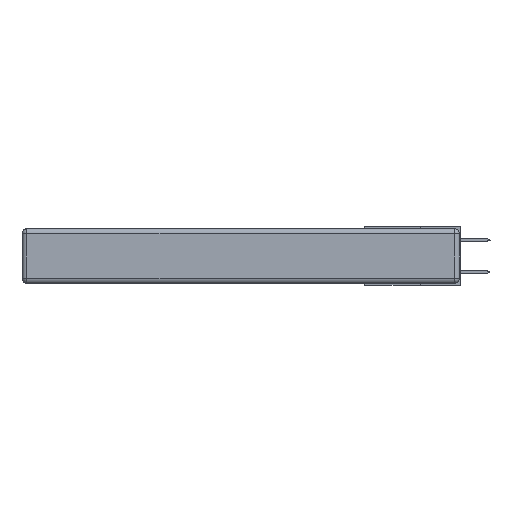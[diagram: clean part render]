
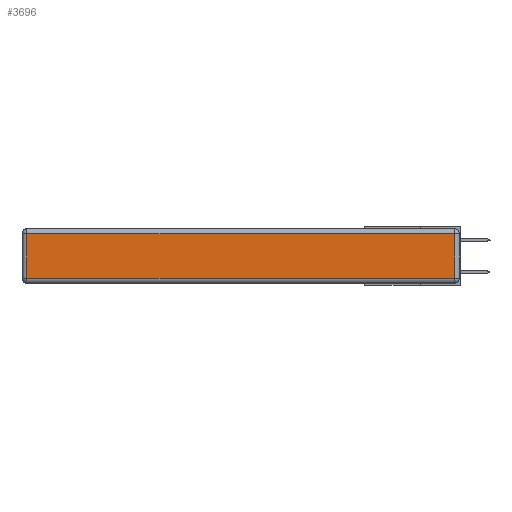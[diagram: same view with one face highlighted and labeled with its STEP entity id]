
A CAD part, left-side view. The second image highlights one B-rep face of the part: STEP entity #3696.
In plain terms, the highlighted planar face has unit normal (-1, 0, 0).
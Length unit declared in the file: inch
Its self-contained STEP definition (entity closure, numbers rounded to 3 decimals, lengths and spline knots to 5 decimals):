
#923 = ORIENTED_EDGE ( 'NONE', *, *, #18820, .T. ) ;
#1797 = EDGE_CURVE ( 'NONE', #11398, #5262, #14673, .T. ) ;
#3696 = ADVANCED_FACE ( 'NONE', ( #9920 ), #11347, .T. ) ;
#5262 = VERTEX_POINT ( 'NONE', #19997 ) ;
#7886 = EDGE_CURVE ( 'NONE', #25701, #11398, #31440, .T. ) ;
#8494 = DIRECTION ( 'NONE',  ( 0., -1., 0. ) ) ;
#9450 = ORIENTED_EDGE ( 'NONE', *, *, #7886, .T. ) ;
#9713 = CARTESIAN_POINT ( 'NONE',  ( 0., 0.03, -0.343 ) ) ;
#9920 = FACE_OUTER_BOUND ( 'NONE', #14431, .T. ) ;
#10403 = DIRECTION ( 'NONE',  ( 0., 1., 0. ) ) ;
#11347 = PLANE ( 'NONE',  #12634 ) ;
#11398 = VERTEX_POINT ( 'NONE', #20326 ) ;
#12035 = CARTESIAN_POINT ( 'NONE',  ( 0., 2.72, -0.343 ) ) ;
#12634 = AXIS2_PLACEMENT_3D ( 'NONE', #31629, #21806, #21584 ) ;
#12856 = ORIENTED_EDGE ( 'NONE', *, *, #13616, .T. ) ;
#13616 = EDGE_CURVE ( 'NONE', #16499, #25701, #19919, .T. ) ;
#14431 = EDGE_LOOP ( 'NONE', ( #923, #12856, #9450, #26499 ) ) ;
#14673 = LINE ( 'NONE', #12035, #27037 ) ;
#15405 = CARTESIAN_POINT ( 'NONE',  ( 0., 2.75, -0.03 ) ) ;
#16043 = CARTESIAN_POINT ( 'NONE',  ( 0., 0.03, -0.313 ) ) ;
#16499 = VERTEX_POINT ( 'NONE', #16043 ) ;
#16637 = DIRECTION ( 'NONE',  ( 0., 0., -1. ) ) ;
#18666 = CARTESIAN_POINT ( 'NONE',  ( 0., 0.03, -0.03 ) ) ;
#18820 = EDGE_CURVE ( 'NONE', #5262, #16499, #31346, .T. ) ;
#19787 = DIRECTION ( 'NONE',  ( 0., 0., 1. ) ) ;
#19919 = LINE ( 'NONE', #9713, #29002 ) ;
#19997 = CARTESIAN_POINT ( 'NONE',  ( 0., 2.72, -0.313 ) ) ;
#20326 = CARTESIAN_POINT ( 'NONE',  ( 0., 2.72, -0.03 ) ) ;
#21584 = DIRECTION ( 'NONE',  ( 0., 0., 1. ) ) ;
#21806 = DIRECTION ( 'NONE',  ( -1., 0., 0. ) ) ;
#21970 = VECTOR ( 'NONE', #10403, 39.37008 ) ;
#22219 = VECTOR ( 'NONE', #8494, 39.37008 ) ;
#25701 = VERTEX_POINT ( 'NONE', #18666 ) ;
#26499 = ORIENTED_EDGE ( 'NONE', *, *, #1797, .T. ) ;
#27037 = VECTOR ( 'NONE', #16637, 39.37008 ) ;
#29002 = VECTOR ( 'NONE', #19787, 39.37008 ) ;
#31346 = LINE ( 'NONE', #31446, #22219 ) ;
#31440 = LINE ( 'NONE', #15405, #21970 ) ;
#31446 = CARTESIAN_POINT ( 'NONE',  ( 0., 0., -0.313 ) ) ;
#31629 = CARTESIAN_POINT ( 'NONE',  ( 0., 0., -0.343 ) ) ;
